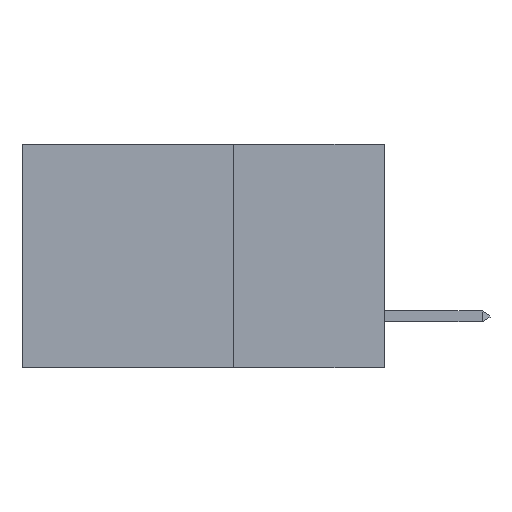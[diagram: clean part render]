
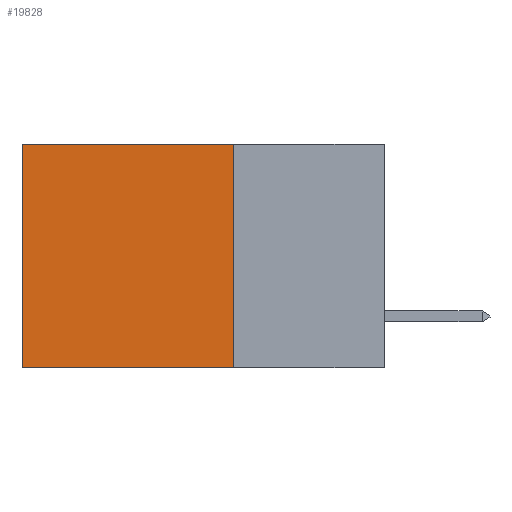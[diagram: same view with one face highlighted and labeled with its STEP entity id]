
A CAD part, left-side view. The second image highlights one B-rep face of the part: STEP entity #19828.
In plain terms, the highlighted planar face has unit normal (-1, 0, 0).
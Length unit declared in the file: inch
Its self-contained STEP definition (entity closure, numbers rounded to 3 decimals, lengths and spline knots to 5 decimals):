
#310 = CARTESIAN_POINT ( 'NONE',  ( 0.2875, 0.6, 0. ) ) ;
#616 = CARTESIAN_POINT ( 'NONE',  ( 0.2875, 0.25, -0.37 ) ) ;
#792 = CARTESIAN_POINT ( 'NONE',  ( 0.2875, 0.6, 0. ) ) ;
#1001 = DIRECTION ( 'NONE',  ( 0., 1., 0. ) ) ;
#1343 = ORIENTED_EDGE ( 'NONE', *, *, #2176, .F. ) ;
#2176 = EDGE_CURVE ( 'NONE', #3590, #11436, #19340, .T. ) ;
#2649 = LINE ( 'NONE', #310, #15018 ) ;
#3293 = EDGE_LOOP ( 'NONE', ( #4494, #4157, #1343, #6002 ) ) ;
#3314 = DIRECTION ( 'NONE',  ( 1., 0., 0. ) ) ;
#3572 = DIRECTION ( 'NONE',  ( 0., 0., -1. ) ) ;
#3590 = VERTEX_POINT ( 'NONE', #10465 ) ;
#4079 = CARTESIAN_POINT ( 'NONE',  ( 0.2875, 0.6, -0.37 ) ) ;
#4157 = ORIENTED_EDGE ( 'NONE', *, *, #10943, .F. ) ;
#4181 = VERTEX_POINT ( 'NONE', #792 ) ;
#4494 = ORIENTED_EDGE ( 'NONE', *, *, #8981, .T. ) ;
#5376 = AXIS2_PLACEMENT_3D ( 'NONE', #13058, #3314, #14616 ) ;
#5571 = VECTOR ( 'NONE', #17451, 39.37008 ) ;
#6002 = ORIENTED_EDGE ( 'NONE', *, *, #15497, .T. ) ;
#6377 = CARTESIAN_POINT ( 'NONE',  ( 0.2875, 0.25, 0. ) ) ;
#6547 = PLANE ( 'NONE',  #5376 ) ;
#8981 = EDGE_CURVE ( 'NONE', #4181, #15261, #2649, .T. ) ;
#9078 = VECTOR ( 'NONE', #1001, 39.37008 ) ;
#10286 = CARTESIAN_POINT ( 'NONE',  ( 0.2875, 0.25, 0. ) ) ;
#10465 = CARTESIAN_POINT ( 'NONE',  ( 0.2875, 0.25, 0. ) ) ;
#10759 = CARTESIAN_POINT ( 'NONE',  ( 0.2875, 0.25, -0.37 ) ) ;
#10943 = EDGE_CURVE ( 'NONE', #11436, #15261, #16937, .T. ) ;
#11142 = VECTOR ( 'NONE', #13732, 39.37008 ) ;
#11436 = VERTEX_POINT ( 'NONE', #616 ) ;
#13058 = CARTESIAN_POINT ( 'NONE',  ( 0.2875, 0.25, 0. ) ) ;
#13732 = DIRECTION ( 'NONE',  ( 0., 0., -1. ) ) ;
#14165 = LINE ( 'NONE', #6377, #5571 ) ;
#14616 = DIRECTION ( 'NONE',  ( 0., 0., -1. ) ) ;
#15018 = VECTOR ( 'NONE', #3572, 39.37008 ) ;
#15261 = VERTEX_POINT ( 'NONE', #4079 ) ;
#15497 = EDGE_CURVE ( 'NONE', #3590, #4181, #14165, .T. ) ;
#16937 = LINE ( 'NONE', #10759, #9078 ) ;
#17451 = DIRECTION ( 'NONE',  ( 0., 1., 0. ) ) ;
#19340 = LINE ( 'NONE', #10286, #11142 ) ;
#19828 = ADVANCED_FACE ( 'NONE', ( #19869 ), #6547, .F. ) ;
#19869 = FACE_OUTER_BOUND ( 'NONE', #3293, .T. ) ;
